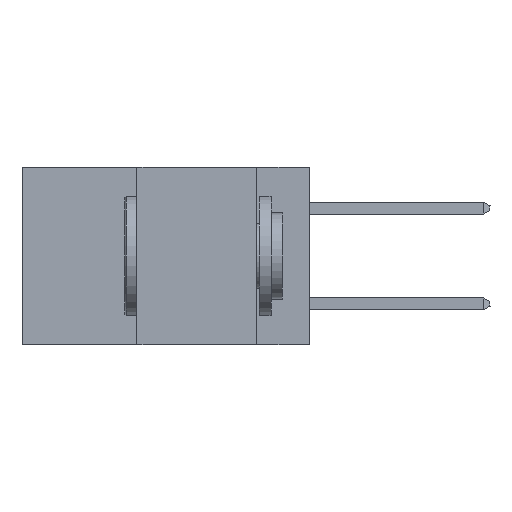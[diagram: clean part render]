
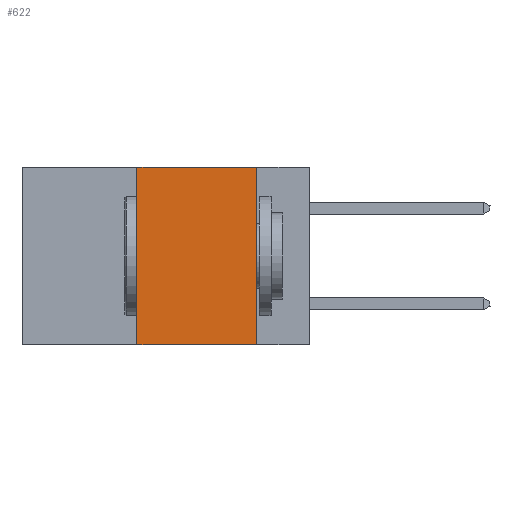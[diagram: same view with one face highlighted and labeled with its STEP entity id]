
A CAD part, left-side view. The second image highlights one B-rep face of the part: STEP entity #622.
In plain terms, the highlighted planar face has unit normal (-1, 0, 0).
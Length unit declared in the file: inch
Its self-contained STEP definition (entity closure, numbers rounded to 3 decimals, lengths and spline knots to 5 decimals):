
#150 = EDGE_CURVE ( 'NONE', #4639, #4360, #4702, .T. ) ;
#622 = ADVANCED_FACE ( 'NONE', ( #18958 ), #18084, .F. ) ;
#1074 = EDGE_LOOP ( 'NONE', ( #10308, #11831, #8406, #21317 ) ) ;
#1234 = AXIS2_PLACEMENT_3D ( 'NONE', #16236, #9119, #14413 ) ;
#1369 = EDGE_CURVE ( 'NONE', #22667, #4465, #9972, .T. ) ;
#1929 = CARTESIAN_POINT ( 'NONE',  ( 0., 0.6, -0.37 ) ) ;
#2767 = CARTESIAN_POINT ( 'NONE',  ( 0., 0.11, 0. ) ) ;
#4360 = VERTEX_POINT ( 'NONE', #2767 ) ;
#4465 = VERTEX_POINT ( 'NONE', #4647 ) ;
#4639 = VERTEX_POINT ( 'NONE', #8729 ) ;
#4647 = CARTESIAN_POINT ( 'NONE',  ( 0., 0.11, -0.37 ) ) ;
#4702 = LINE ( 'NONE', #9004, #17621 ) ;
#4913 = EDGE_CURVE ( 'NONE', #22667, #4639, #12845, .T. ) ;
#5547 = CARTESIAN_POINT ( 'NONE',  ( 0., 0.36, 0. ) ) ;
#5605 = DIRECTION ( 'NONE',  ( 0., -1., 0. ) ) ;
#6397 = VECTOR ( 'NONE', #12289, 39.37008 ) ;
#6717 = DIRECTION ( 'NONE',  ( 0., 0., -1. ) ) ;
#7897 = EDGE_CURVE ( 'NONE', #4360, #4465, #14238, .T. ) ;
#8406 = ORIENTED_EDGE ( 'NONE', *, *, #4913, .F. ) ;
#8729 = CARTESIAN_POINT ( 'NONE',  ( 0., 0.36, 0. ) ) ;
#9004 = CARTESIAN_POINT ( 'NONE',  ( 0., 0.6, 0. ) ) ;
#9119 = DIRECTION ( 'NONE',  ( 1., 0., 0. ) ) ;
#9568 = VECTOR ( 'NONE', #6717, 39.37008 ) ;
#9972 = LINE ( 'NONE', #1929, #6397 ) ;
#10308 = ORIENTED_EDGE ( 'NONE', *, *, #7897, .F. ) ;
#11831 = ORIENTED_EDGE ( 'NONE', *, *, #150, .F. ) ;
#12289 = DIRECTION ( 'NONE',  ( 0., -1., 0. ) ) ;
#12845 = LINE ( 'NONE', #5547, #20460 ) ;
#14238 = LINE ( 'NONE', #21899, #9568 ) ;
#14413 = DIRECTION ( 'NONE',  ( 0., 0., -1. ) ) ;
#15574 = CARTESIAN_POINT ( 'NONE',  ( 0., 0.36, -0.37 ) ) ;
#16236 = CARTESIAN_POINT ( 'NONE',  ( 0., 0.6, 0. ) ) ;
#17604 = DIRECTION ( 'NONE',  ( 0., 0., 1. ) ) ;
#17621 = VECTOR ( 'NONE', #5605, 39.37008 ) ;
#18084 = PLANE ( 'NONE',  #1234 ) ;
#18958 = FACE_OUTER_BOUND ( 'NONE', #1074, .T. ) ;
#20460 = VECTOR ( 'NONE', #17604, 39.37008 ) ;
#21317 = ORIENTED_EDGE ( 'NONE', *, *, #1369, .T. ) ;
#21899 = CARTESIAN_POINT ( 'NONE',  ( 0., 0.11, 0. ) ) ;
#22667 = VERTEX_POINT ( 'NONE', #15574 ) ;
